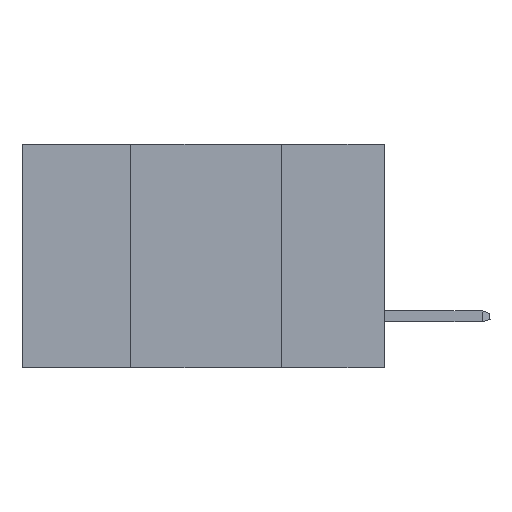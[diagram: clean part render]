
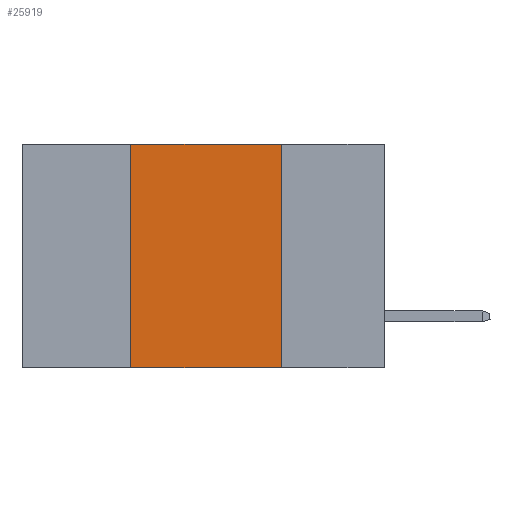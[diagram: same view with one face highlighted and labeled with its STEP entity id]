
A CAD part, left-side view. The second image highlights one B-rep face of the part: STEP entity #25919.
In plain terms, the highlighted planar face has unit normal (-1, 0, 0).
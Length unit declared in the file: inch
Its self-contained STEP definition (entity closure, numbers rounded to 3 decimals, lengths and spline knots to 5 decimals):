
#828 = EDGE_CURVE ( 'NONE', #16763, #8365, #11521, .T. ) ;
#1485 = CARTESIAN_POINT ( 'NONE',  ( 0., 0.6, 0. ) ) ;
#2056 = ORIENTED_EDGE ( 'NONE', *, *, #14177, .F. ) ;
#2391 = CARTESIAN_POINT ( 'NONE',  ( 0., 0.17, 0. ) ) ;
#3194 = DIRECTION ( 'NONE',  ( 0., -1., 0. ) ) ;
#4669 = ORIENTED_EDGE ( 'NONE', *, *, #16214, .T. ) ;
#4675 = CARTESIAN_POINT ( 'NONE',  ( 0., 0.42, 0. ) ) ;
#5127 = CARTESIAN_POINT ( 'NONE',  ( 0., 0.42, -0.37 ) ) ;
#7168 = VECTOR ( 'NONE', #23234, 39.37008 ) ;
#7221 = CARTESIAN_POINT ( 'NONE',  ( 0., 0.6, -0.37 ) ) ;
#8365 = VERTEX_POINT ( 'NONE', #11938 ) ;
#9197 = DIRECTION ( 'NONE',  ( 0., 0., -1. ) ) ;
#9386 = DIRECTION ( 'NONE',  ( 1., 0., 0. ) ) ;
#10406 = FACE_OUTER_BOUND ( 'NONE', #15837, .T. ) ;
#11434 = CARTESIAN_POINT ( 'NONE',  ( 0., 0.6, 0. ) ) ;
#11474 = VERTEX_POINT ( 'NONE', #2391 ) ;
#11521 = LINE ( 'NONE', #4675, #14895 ) ;
#11713 = ORIENTED_EDGE ( 'NONE', *, *, #16292, .F. ) ;
#11938 = CARTESIAN_POINT ( 'NONE',  ( 0., 0.42, 0. ) ) ;
#14177 = EDGE_CURVE ( 'NONE', #11474, #21751, #17856, .T. ) ;
#14811 = CARTESIAN_POINT ( 'NONE',  ( 0., 0.17, 0. ) ) ;
#14895 = VECTOR ( 'NONE', #20691, 39.37008 ) ;
#15837 = EDGE_LOOP ( 'NONE', ( #2056, #11713, #27229, #4669 ) ) ;
#16214 = EDGE_CURVE ( 'NONE', #16763, #21751, #24089, .T. ) ;
#16292 = EDGE_CURVE ( 'NONE', #8365, #11474, #23672, .T. ) ;
#16763 = VERTEX_POINT ( 'NONE', #5127 ) ;
#17311 = VECTOR ( 'NONE', #24893, 39.37008 ) ;
#17856 = LINE ( 'NONE', #14811, #7168 ) ;
#19707 = VECTOR ( 'NONE', #3194, 39.37008 ) ;
#20691 = DIRECTION ( 'NONE',  ( 0., 0., 1. ) ) ;
#21751 = VERTEX_POINT ( 'NONE', #22752 ) ;
#22752 = CARTESIAN_POINT ( 'NONE',  ( 0., 0.17, -0.37 ) ) ;
#23234 = DIRECTION ( 'NONE',  ( 0., 0., -1. ) ) ;
#23672 = LINE ( 'NONE', #1485, #17311 ) ;
#24089 = LINE ( 'NONE', #7221, #19707 ) ;
#24447 = PLANE ( 'NONE',  #25439 ) ;
#24893 = DIRECTION ( 'NONE',  ( 0., -1., 0. ) ) ;
#25439 = AXIS2_PLACEMENT_3D ( 'NONE', #11434, #9386, #9197 ) ;
#25919 = ADVANCED_FACE ( 'NONE', ( #10406 ), #24447, .F. ) ;
#27229 = ORIENTED_EDGE ( 'NONE', *, *, #828, .F. ) ;
